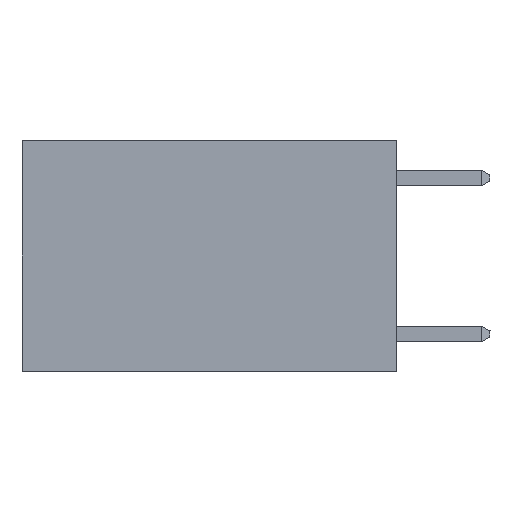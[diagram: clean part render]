
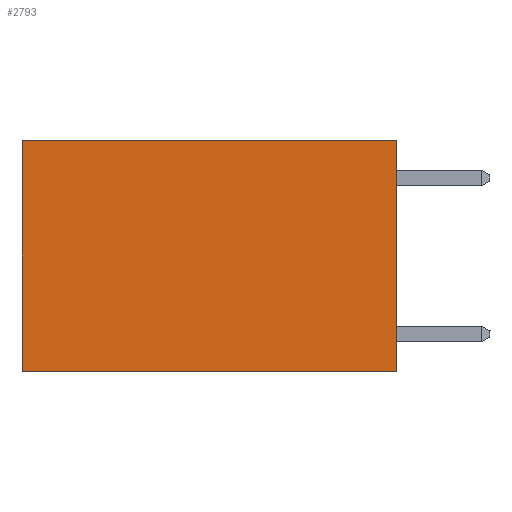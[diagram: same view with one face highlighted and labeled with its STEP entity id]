
A CAD part, left-side view. The second image highlights one B-rep face of the part: STEP entity #2793.
In plain terms, the highlighted planar face has unit normal (-1, 0, 0).
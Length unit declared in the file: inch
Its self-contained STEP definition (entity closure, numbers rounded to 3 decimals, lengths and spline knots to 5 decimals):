
#365 = EDGE_CURVE ( 'NONE', #4822, #8907, #7984, .T. ) ;
#613 = CARTESIAN_POINT ( 'NONE',  ( 0.2625, 0.6, 0. ) ) ;
#1110 = CARTESIAN_POINT ( 'NONE',  ( 0.2625, 0.6, 0. ) ) ;
#2114 = CARTESIAN_POINT ( 'NONE',  ( 0.2625, 0., 0. ) ) ;
#2793 = ADVANCED_FACE ( 'NONE', ( #3554 ), #7972, .F. ) ;
#2859 = VECTOR ( 'NONE', #8070, 39.37008 ) ;
#2895 = CARTESIAN_POINT ( 'NONE',  ( 0.2625, 0., 0. ) ) ;
#3395 = VECTOR ( 'NONE', #7796, 39.37008 ) ;
#3554 = FACE_OUTER_BOUND ( 'NONE', #6317, .T. ) ;
#3663 = EDGE_CURVE ( 'NONE', #4822, #8118, #6994, .T. ) ;
#3911 = CARTESIAN_POINT ( 'NONE',  ( 0.2625, 0.6, -0.37 ) ) ;
#4166 = CARTESIAN_POINT ( 'NONE',  ( 0.2625, 0., -0.37 ) ) ;
#4291 = DIRECTION ( 'NONE',  ( 0., 0., -1. ) ) ;
#4822 = VERTEX_POINT ( 'NONE', #2114 ) ;
#5026 = DIRECTION ( 'NONE',  ( 0., 0., -1. ) ) ;
#5194 = VECTOR ( 'NONE', #5026, 39.37008 ) ;
#5720 = ORIENTED_EDGE ( 'NONE', *, *, #8301, .T. ) ;
#5862 = VECTOR ( 'NONE', #4291, 39.37008 ) ;
#5867 = ORIENTED_EDGE ( 'NONE', *, *, #8742, .F. ) ;
#5870 = ORIENTED_EDGE ( 'NONE', *, *, #365, .F. ) ;
#5888 = ORIENTED_EDGE ( 'NONE', *, *, #3663, .T. ) ;
#6122 = DIRECTION ( 'NONE',  ( 0., 0., -1. ) ) ;
#6161 = DIRECTION ( 'NONE',  ( 1., 0., 0. ) ) ;
#6210 = AXIS2_PLACEMENT_3D ( 'NONE', #7840, #6161, #6122 ) ;
#6317 = EDGE_LOOP ( 'NONE', ( #5720, #5867, #5870, #5888 ) ) ;
#6511 = CARTESIAN_POINT ( 'NONE',  ( 0.2625, 0., -0.37 ) ) ;
#6994 = LINE ( 'NONE', #2895, #2859 ) ;
#7796 = DIRECTION ( 'NONE',  ( 0., 1., 0. ) ) ;
#7840 = CARTESIAN_POINT ( 'NONE',  ( 0.2625, 0., 0. ) ) ;
#7972 = PLANE ( 'NONE',  #6210 ) ;
#7984 = LINE ( 'NONE', #9182, #5862 ) ;
#7994 = VERTEX_POINT ( 'NONE', #3911 ) ;
#8070 = DIRECTION ( 'NONE',  ( 0., 1., 0. ) ) ;
#8118 = VERTEX_POINT ( 'NONE', #1110 ) ;
#8301 = EDGE_CURVE ( 'NONE', #8118, #7994, #9208, .T. ) ;
#8742 = EDGE_CURVE ( 'NONE', #8907, #7994, #9347, .T. ) ;
#8907 = VERTEX_POINT ( 'NONE', #6511 ) ;
#9182 = CARTESIAN_POINT ( 'NONE',  ( 0.2625, 0., 0. ) ) ;
#9208 = LINE ( 'NONE', #613, #5194 ) ;
#9347 = LINE ( 'NONE', #4166, #3395 ) ;
